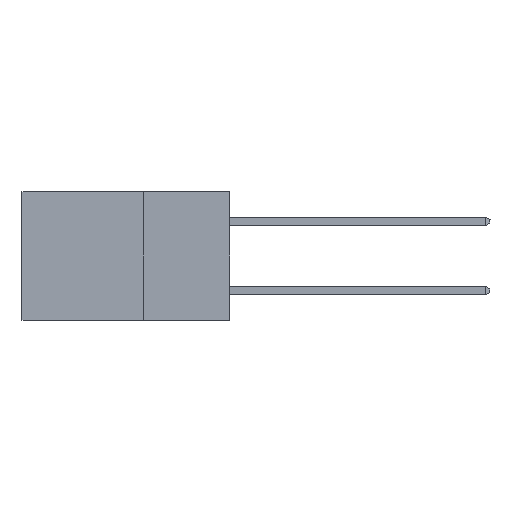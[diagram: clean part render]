
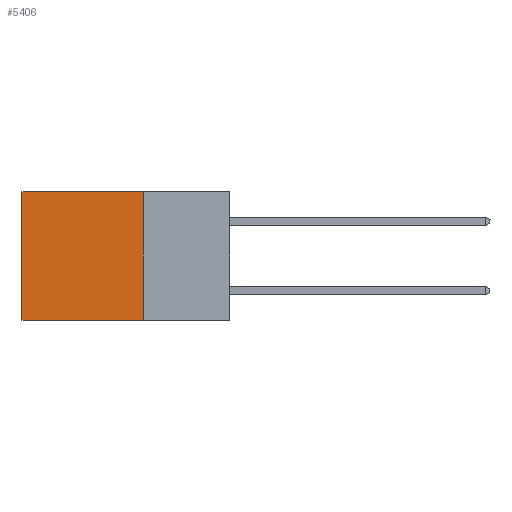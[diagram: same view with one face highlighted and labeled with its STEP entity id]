
A CAD part, left-side view. The second image highlights one B-rep face of the part: STEP entity #5406.
In plain terms, the highlighted planar face has unit normal (-1, 0, 0).
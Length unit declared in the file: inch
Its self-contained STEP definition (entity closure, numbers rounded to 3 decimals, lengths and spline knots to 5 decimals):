
#240 = DIRECTION ( 'NONE',  ( 0., 0., -1. ) ) ;
#875 = VERTEX_POINT ( 'NONE', #6625 ) ;
#912 = VECTOR ( 'NONE', #240, 39.37008 ) ;
#1546 = ORIENTED_EDGE ( 'NONE', *, *, #6944, .T. ) ;
#1579 = DIRECTION ( 'NONE',  ( 1., 0., 0. ) ) ;
#2484 = CARTESIAN_POINT ( 'NONE',  ( 0.298, 0.25, 0. ) ) ;
#2598 = PLANE ( 'NONE',  #10483 ) ;
#3065 = CARTESIAN_POINT ( 'NONE',  ( 0.298, 0.25, 0. ) ) ;
#3356 = DIRECTION ( 'NONE',  ( 0., 0., -1. ) ) ;
#3523 = CARTESIAN_POINT ( 'NONE',  ( 0.298, 0.25, 0. ) ) ;
#3755 = CARTESIAN_POINT ( 'NONE',  ( 0.298, 0.6, 0. ) ) ;
#3756 = EDGE_CURVE ( 'NONE', #7120, #8859, #10959, .T. ) ;
#5406 = ADVANCED_FACE ( 'NONE', ( #6323 ), #2598, .F. ) ;
#5539 = CARTESIAN_POINT ( 'NONE',  ( 0.298, 0.25, 0. ) ) ;
#5916 = DIRECTION ( 'NONE',  ( 0., 1., 0. ) ) ;
#5988 = VERTEX_POINT ( 'NONE', #3065 ) ;
#6218 = LINE ( 'NONE', #9379, #9911 ) ;
#6305 = ORIENTED_EDGE ( 'NONE', *, *, #11225, .F. ) ;
#6323 = FACE_OUTER_BOUND ( 'NONE', #9408, .T. ) ;
#6412 = VECTOR ( 'NONE', #10464, 39.37008 ) ;
#6625 = CARTESIAN_POINT ( 'NONE',  ( 0.298, 0.25, -0.37 ) ) ;
#6944 = EDGE_CURVE ( 'NONE', #5988, #7120, #10376, .T. ) ;
#7120 = VERTEX_POINT ( 'NONE', #7407 ) ;
#7407 = CARTESIAN_POINT ( 'NONE',  ( 0.298, 0.6, 0. ) ) ;
#7574 = CARTESIAN_POINT ( 'NONE',  ( 0.298, 0.6, -0.37 ) ) ;
#8030 = ORIENTED_EDGE ( 'NONE', *, *, #3756, .T. ) ;
#8219 = VECTOR ( 'NONE', #10644, 39.37008 ) ;
#8859 = VERTEX_POINT ( 'NONE', #7574 ) ;
#9379 = CARTESIAN_POINT ( 'NONE',  ( 0.298, 0.25, -0.37 ) ) ;
#9408 = EDGE_LOOP ( 'NONE', ( #8030, #10840, #6305, #1546 ) ) ;
#9511 = EDGE_CURVE ( 'NONE', #875, #8859, #6218, .T. ) ;
#9911 = VECTOR ( 'NONE', #5916, 39.37008 ) ;
#9997 = LINE ( 'NONE', #5539, #8219 ) ;
#10376 = LINE ( 'NONE', #3523, #6412 ) ;
#10464 = DIRECTION ( 'NONE',  ( 0., 1., 0. ) ) ;
#10483 = AXIS2_PLACEMENT_3D ( 'NONE', #2484, #1579, #3356 ) ;
#10644 = DIRECTION ( 'NONE',  ( 0., 0., -1. ) ) ;
#10840 = ORIENTED_EDGE ( 'NONE', *, *, #9511, .F. ) ;
#10959 = LINE ( 'NONE', #3755, #912 ) ;
#11225 = EDGE_CURVE ( 'NONE', #5988, #875, #9997, .T. ) ;
